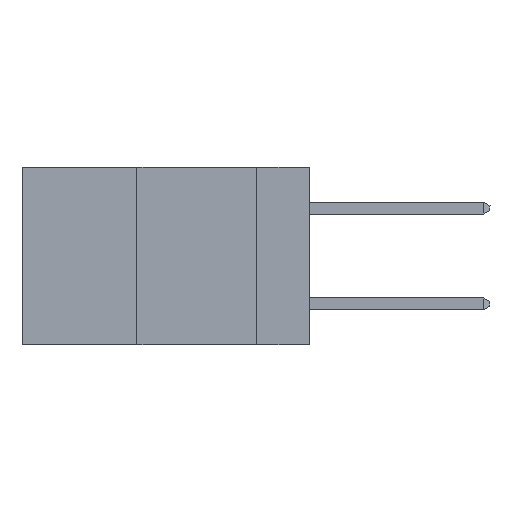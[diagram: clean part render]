
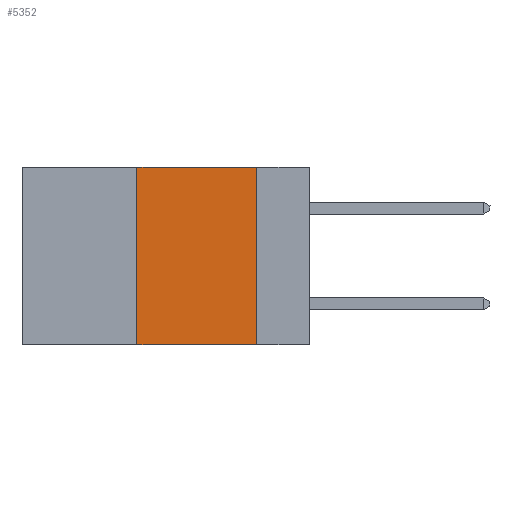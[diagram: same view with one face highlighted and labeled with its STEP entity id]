
A CAD part, left-side view. The second image highlights one B-rep face of the part: STEP entity #5352.
In plain terms, the highlighted planar face has unit normal (-1, 0, 0).
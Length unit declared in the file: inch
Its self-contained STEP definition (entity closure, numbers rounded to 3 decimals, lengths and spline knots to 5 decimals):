
#94 = DIRECTION ( 'NONE',  ( 0., 0., -1. ) ) ;
#358 = LINE ( 'NONE', #13709, #3195 ) ;
#449 = CARTESIAN_POINT ( 'NONE',  ( 0., 0.11, 0. ) ) ;
#1025 = VERTEX_POINT ( 'NONE', #10838 ) ;
#1460 = CARTESIAN_POINT ( 'NONE',  ( 0., 0.36, 0. ) ) ;
#1489 = EDGE_CURVE ( 'NONE', #6551, #15323, #8729, .T. ) ;
#1513 = VERTEX_POINT ( 'NONE', #1460 ) ;
#2376 = CARTESIAN_POINT ( 'NONE',  ( 0., 0.6, 0. ) ) ;
#2979 = ORIENTED_EDGE ( 'NONE', *, *, #1489, .F. ) ;
#3054 = ORIENTED_EDGE ( 'NONE', *, *, #4903, .F. ) ;
#3090 = LINE ( 'NONE', #2376, #9072 ) ;
#3188 = ORIENTED_EDGE ( 'NONE', *, *, #9771, .F. ) ;
#3195 = VECTOR ( 'NONE', #3258, 39.37008 ) ;
#3258 = DIRECTION ( 'NONE',  ( 0., 0., 1. ) ) ;
#3330 = EDGE_CURVE ( 'NONE', #1025, #15323, #7592, .T. ) ;
#3335 = ORIENTED_EDGE ( 'NONE', *, *, #3330, .T. ) ;
#3765 = DIRECTION ( 'NONE',  ( 0., -1., 0. ) ) ;
#4368 = VECTOR ( 'NONE', #12541, 39.37008 ) ;
#4903 = EDGE_CURVE ( 'NONE', #1513, #6551, #3090, .T. ) ;
#5352 = ADVANCED_FACE ( 'NONE', ( #10673 ), #13897, .F. ) ;
#6551 = VERTEX_POINT ( 'NONE', #15290 ) ;
#7592 = LINE ( 'NONE', #10306, #4368 ) ;
#8311 = DIRECTION ( 'NONE',  ( 0., 0., -1. ) ) ;
#8378 = VECTOR ( 'NONE', #94, 39.37008 ) ;
#8612 = EDGE_LOOP ( 'NONE', ( #2979, #3054, #3188, #3335 ) ) ;
#8729 = LINE ( 'NONE', #449, #8378 ) ;
#9072 = VECTOR ( 'NONE', #3765, 39.37008 ) ;
#9393 = CARTESIAN_POINT ( 'NONE',  ( 0., 0.6, 0. ) ) ;
#9771 = EDGE_CURVE ( 'NONE', #1025, #1513, #358, .T. ) ;
#10306 = CARTESIAN_POINT ( 'NONE',  ( 0., 0.6, -0.37 ) ) ;
#10673 = FACE_OUTER_BOUND ( 'NONE', #8612, .T. ) ;
#10838 = CARTESIAN_POINT ( 'NONE',  ( 0., 0.36, -0.37 ) ) ;
#12541 = DIRECTION ( 'NONE',  ( 0., -1., 0. ) ) ;
#13709 = CARTESIAN_POINT ( 'NONE',  ( 0., 0.36, 0. ) ) ;
#13897 = PLANE ( 'NONE',  #14686 ) ;
#14398 = CARTESIAN_POINT ( 'NONE',  ( 0., 0.11, -0.37 ) ) ;
#14686 = AXIS2_PLACEMENT_3D ( 'NONE', #9393, #15084, #8311 ) ;
#15084 = DIRECTION ( 'NONE',  ( 1., 0., 0. ) ) ;
#15290 = CARTESIAN_POINT ( 'NONE',  ( 0., 0.11, 0. ) ) ;
#15323 = VERTEX_POINT ( 'NONE', #14398 ) ;
